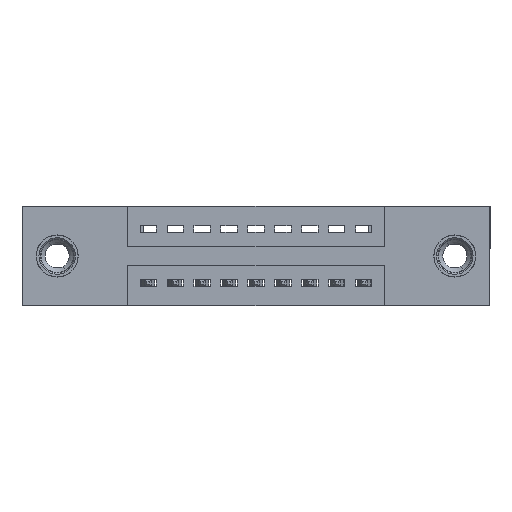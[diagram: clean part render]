
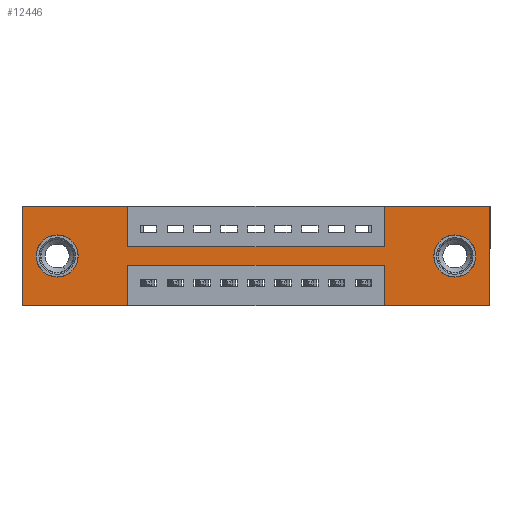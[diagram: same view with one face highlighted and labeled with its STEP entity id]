
A CAD part, front view. The second image highlights one B-rep face of the part: STEP entity #12446.
In plain terms, the highlighted planar face has unit normal (0, -1, 0).
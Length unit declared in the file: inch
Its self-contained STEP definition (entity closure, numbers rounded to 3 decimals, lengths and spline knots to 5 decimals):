
#334 = LINE ( 'NONE', #2685, #6698 ) ;
#385 = ORIENTED_EDGE ( 'NONE', *, *, #4710, .F. ) ;
#691 = CARTESIAN_POINT ( 'NONE',  ( 0.13, 0., -0.263 ) ) ;
#692 = DIRECTION ( 'NONE',  ( -1., 0., 0. ) ) ;
#784 = AXIS2_PLACEMENT_3D ( 'NONE', #1007, #10207, #7212 ) ;
#808 = CARTESIAN_POINT ( 'NONE',  ( 0., 0., 0. ) ) ;
#924 = LINE ( 'NONE', #11011, #5824 ) ;
#981 = VECTOR ( 'NONE', #4509, 39.37008 ) ;
#1007 = CARTESIAN_POINT ( 'NONE',  ( 0., 0., -0.37 ) ) ;
#1125 = CARTESIAN_POINT ( 'NONE',  ( 0., 0., 0. ) ) ;
#1272 = VERTEX_POINT ( 'NONE', #8957 ) ;
#1360 = CIRCLE ( 'NONE', #1492, 0.078 ) ;
#1441 = EDGE_CURVE ( 'NONE', #12947, #3797, #3608, .T. ) ;
#1492 = AXIS2_PLACEMENT_3D ( 'NONE', #10740, #10833, #8743 ) ;
#1558 = DIRECTION ( 'NONE',  ( 0., 0., -1. ) ) ;
#1572 = DIRECTION ( 'NONE',  ( 0., 0., 1. ) ) ;
#1639 = LINE ( 'NONE', #11636, #981 ) ;
#1731 = ORIENTED_EDGE ( 'NONE', *, *, #2681, .F. ) ;
#1738 = VECTOR ( 'NONE', #6974, 39.37008 ) ;
#1803 = VERTEX_POINT ( 'NONE', #6123 ) ;
#1842 = LINE ( 'NONE', #9720, #3478 ) ;
#1892 = LINE ( 'NONE', #4767, #5170 ) ;
#2051 = PLANE ( 'NONE',  #784 ) ;
#2267 = LINE ( 'NONE', #2532, #9526 ) ;
#2298 = DIRECTION ( 'NONE',  ( 0., 0., 1. ) ) ;
#2302 = CARTESIAN_POINT ( 'NONE',  ( 0.3925, 0., -0.37 ) ) ;
#2353 = CIRCLE ( 'NONE', #8984, 0.078 ) ;
#2532 = CARTESIAN_POINT ( 'NONE',  ( 1.3425, 0., -0.37 ) ) ;
#2676 = CARTESIAN_POINT ( 'NONE',  ( 1.605, 0., -0.185 ) ) ;
#2681 = EDGE_CURVE ( 'NONE', #8704, #9898, #334, .T. ) ;
#2685 = CARTESIAN_POINT ( 'NONE',  ( 0.3925, 0., -0.37 ) ) ;
#2840 = ORIENTED_EDGE ( 'NONE', *, *, #13371, .F. ) ;
#2841 = CARTESIAN_POINT ( 'NONE',  ( 1.735, 0., 0. ) ) ;
#2896 = EDGE_CURVE ( 'NONE', #10257, #7675, #13296, .T. ) ;
#2903 = DIRECTION ( 'NONE',  ( 0., 0., 1. ) ) ;
#2932 = CARTESIAN_POINT ( 'NONE',  ( 1.605, 0., -0.107 ) ) ;
#3339 = DIRECTION ( 'NONE',  ( 0., 0., -1. ) ) ;
#3436 = VECTOR ( 'NONE', #12733, 39.37008 ) ;
#3478 = VECTOR ( 'NONE', #1558, 39.37008 ) ;
#3608 = CIRCLE ( 'NONE', #11707, 0.078 ) ;
#3704 = VERTEX_POINT ( 'NONE', #6932 ) ;
#3776 = LINE ( 'NONE', #6615, #3436 ) ;
#3797 = VERTEX_POINT ( 'NONE', #5947 ) ;
#3839 = VERTEX_POINT ( 'NONE', #8121 ) ;
#4082 = ORIENTED_EDGE ( 'NONE', *, *, #8666, .F. ) ;
#4178 = FACE_BOUND ( 'NONE', #4181, .T. ) ;
#4181 = EDGE_LOOP ( 'NONE', ( #12147, #12613 ) ) ;
#4392 = EDGE_CURVE ( 'NONE', #5944, #8704, #7937, .T. ) ;
#4408 = LINE ( 'NONE', #808, #9525 ) ;
#4411 = EDGE_CURVE ( 'NONE', #3839, #10896, #3776, .T. ) ;
#4448 = EDGE_CURVE ( 'NONE', #9898, #3704, #1639, .T. ) ;
#4477 = EDGE_LOOP ( 'NONE', ( #1731, #12699, #385, #7774, #12671, #5190, #6355, #4082, #2840, #12896, #13380, #10411 ) ) ;
#4490 = CARTESIAN_POINT ( 'NONE',  ( 0.3925, 0., -0.22 ) ) ;
#4509 = DIRECTION ( 'NONE',  ( -1., 0., 0. ) ) ;
#4682 = ORIENTED_EDGE ( 'NONE', *, *, #11903, .T. ) ;
#4710 = EDGE_CURVE ( 'NONE', #11874, #5944, #2267, .T. ) ;
#4767 = CARTESIAN_POINT ( 'NONE',  ( 0., 0., -0.37 ) ) ;
#4922 = DIRECTION ( 'NONE',  ( 0., 1., 0. ) ) ;
#5128 = FACE_BOUND ( 'NONE', #9958, .T. ) ;
#5139 = CARTESIAN_POINT ( 'NONE',  ( 1.3425, 0., -0.22 ) ) ;
#5170 = VECTOR ( 'NONE', #692, 39.37008 ) ;
#5190 = ORIENTED_EDGE ( 'NONE', *, *, #4411, .F. ) ;
#5260 = VECTOR ( 'NONE', #7839, 39.37008 ) ;
#5419 = CARTESIAN_POINT ( 'NONE',  ( 0.3925, 0., -0.22 ) ) ;
#5654 = VERTEX_POINT ( 'NONE', #7138 ) ;
#5824 = VECTOR ( 'NONE', #12046, 39.37008 ) ;
#5944 = VERTEX_POINT ( 'NONE', #5139 ) ;
#5947 = CARTESIAN_POINT ( 'NONE',  ( 0.13, 0., -0.107 ) ) ;
#5952 = DIRECTION ( 'NONE',  ( 0., 0., -1. ) ) ;
#6123 = CARTESIAN_POINT ( 'NONE',  ( 1.735, 0., -0.37 ) ) ;
#6355 = ORIENTED_EDGE ( 'NONE', *, *, #10820, .F. ) ;
#6592 = CARTESIAN_POINT ( 'NONE',  ( 0.3925, 0., -0.15 ) ) ;
#6615 = CARTESIAN_POINT ( 'NONE',  ( 0., 0., 0. ) ) ;
#6698 = VECTOR ( 'NONE', #9248, 39.37008 ) ;
#6717 = EDGE_CURVE ( 'NONE', #10421, #5654, #12549, .T. ) ;
#6860 = LINE ( 'NONE', #6957, #5260 ) ;
#6908 = CARTESIAN_POINT ( 'NONE',  ( 0.13, 0., -0.185 ) ) ;
#6932 = CARTESIAN_POINT ( 'NONE',  ( 0., 0., -0.37 ) ) ;
#6957 = CARTESIAN_POINT ( 'NONE',  ( 0.3925, 0., -0.15 ) ) ;
#6974 = DIRECTION ( 'NONE',  ( 1., 0., 0. ) ) ;
#7138 = CARTESIAN_POINT ( 'NONE',  ( 0.3925, 0., 0. ) ) ;
#7212 = DIRECTION ( 'NONE',  ( 0., 0., -1. ) ) ;
#7393 = DIRECTION ( 'NONE',  ( 0., 0., 1. ) ) ;
#7675 = VERTEX_POINT ( 'NONE', #12763 ) ;
#7774 = ORIENTED_EDGE ( 'NONE', *, *, #11332, .F. ) ;
#7839 = DIRECTION ( 'NONE',  ( 1., 0., 0. ) ) ;
#7937 = LINE ( 'NONE', #5419, #8245 ) ;
#7955 = EDGE_CURVE ( 'NONE', #10896, #1803, #12042, .T. ) ;
#8121 = CARTESIAN_POINT ( 'NONE',  ( 1.3425, 0., 0. ) ) ;
#8245 = VECTOR ( 'NONE', #10691, 39.37008 ) ;
#8666 = EDGE_CURVE ( 'NONE', #9311, #1272, #6860, .T. ) ;
#8704 = VERTEX_POINT ( 'NONE', #4490 ) ;
#8743 = DIRECTION ( 'NONE',  ( 0., 0., -1. ) ) ;
#8957 = CARTESIAN_POINT ( 'NONE',  ( 1.3425, 0., -0.15 ) ) ;
#8984 = AXIS2_PLACEMENT_3D ( 'NONE', #6908, #12507, #2298 ) ;
#9248 = DIRECTION ( 'NONE',  ( 0., 0., -1. ) ) ;
#9271 = CARTESIAN_POINT ( 'NONE',  ( 0., 0., 0. ) ) ;
#9311 = VERTEX_POINT ( 'NONE', #6592 ) ;
#9488 = DIRECTION ( 'NONE',  ( 0., 1., 0. ) ) ;
#9525 = VECTOR ( 'NONE', #2903, 39.37008 ) ;
#9526 = VECTOR ( 'NONE', #1572, 39.37008 ) ;
#9536 = CARTESIAN_POINT ( 'NONE',  ( 1.3425, 0., -0.37 ) ) ;
#9720 = CARTESIAN_POINT ( 'NONE',  ( 0.3925, 0., 0. ) ) ;
#9742 = EDGE_CURVE ( 'NONE', #3704, #10421, #4408, .T. ) ;
#9898 = VERTEX_POINT ( 'NONE', #2302 ) ;
#9958 = EDGE_LOOP ( 'NONE', ( #4682, #10870 ) ) ;
#10207 = DIRECTION ( 'NONE',  ( 0., -1., 0. ) ) ;
#10257 = VERTEX_POINT ( 'NONE', #2932 ) ;
#10411 = ORIENTED_EDGE ( 'NONE', *, *, #4448, .F. ) ;
#10421 = VERTEX_POINT ( 'NONE', #9271 ) ;
#10575 = CARTESIAN_POINT ( 'NONE',  ( 0.13, 0., -0.185 ) ) ;
#10691 = DIRECTION ( 'NONE',  ( -1., 0., 0. ) ) ;
#10740 = CARTESIAN_POINT ( 'NONE',  ( 1.605, 0., -0.185 ) ) ;
#10742 = VECTOR ( 'NONE', #3339, 39.37008 ) ;
#10820 = EDGE_CURVE ( 'NONE', #1272, #3839, #924, .T. ) ;
#10833 = DIRECTION ( 'NONE',  ( 0., 1., 0. ) ) ;
#10870 = ORIENTED_EDGE ( 'NONE', *, *, #1441, .T. ) ;
#10896 = VERTEX_POINT ( 'NONE', #2841 ) ;
#11011 = CARTESIAN_POINT ( 'NONE',  ( 1.3425, 0., 0. ) ) ;
#11332 = EDGE_CURVE ( 'NONE', #1803, #11874, #1892, .T. ) ;
#11471 = AXIS2_PLACEMENT_3D ( 'NONE', #2676, #4922, #5952 ) ;
#11572 = CARTESIAN_POINT ( 'NONE',  ( 1.735, 0., 0. ) ) ;
#11636 = CARTESIAN_POINT ( 'NONE',  ( 0., 0., -0.37 ) ) ;
#11707 = AXIS2_PLACEMENT_3D ( 'NONE', #10575, #9488, #7393 ) ;
#11874 = VERTEX_POINT ( 'NONE', #9536 ) ;
#11903 = EDGE_CURVE ( 'NONE', #3797, #12947, #2353, .T. ) ;
#12042 = LINE ( 'NONE', #11572, #10742 ) ;
#12046 = DIRECTION ( 'NONE',  ( 0., 0., 1. ) ) ;
#12147 = ORIENTED_EDGE ( 'NONE', *, *, #2896, .T. ) ;
#12348 = FACE_OUTER_BOUND ( 'NONE', #4477, .T. ) ;
#12446 = ADVANCED_FACE ( 'NONE', ( #4178, #5128, #12348 ), #2051, .T. ) ;
#12507 = DIRECTION ( 'NONE',  ( 0., 1., 0. ) ) ;
#12549 = LINE ( 'NONE', #1125, #1738 ) ;
#12600 = EDGE_CURVE ( 'NONE', #7675, #10257, #1360, .T. ) ;
#12613 = ORIENTED_EDGE ( 'NONE', *, *, #12600, .T. ) ;
#12671 = ORIENTED_EDGE ( 'NONE', *, *, #7955, .F. ) ;
#12699 = ORIENTED_EDGE ( 'NONE', *, *, #4392, .F. ) ;
#12733 = DIRECTION ( 'NONE',  ( 1., 0., 0. ) ) ;
#12763 = CARTESIAN_POINT ( 'NONE',  ( 1.605, 0., -0.263 ) ) ;
#12896 = ORIENTED_EDGE ( 'NONE', *, *, #6717, .F. ) ;
#12947 = VERTEX_POINT ( 'NONE', #691 ) ;
#13296 = CIRCLE ( 'NONE', #11471, 0.078 ) ;
#13371 = EDGE_CURVE ( 'NONE', #5654, #9311, #1842, .T. ) ;
#13380 = ORIENTED_EDGE ( 'NONE', *, *, #9742, .F. ) ;
